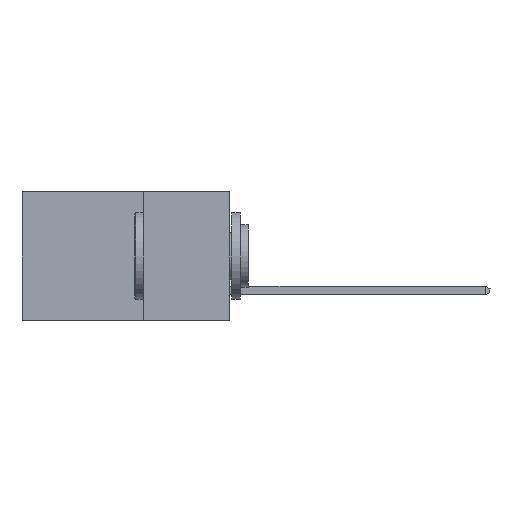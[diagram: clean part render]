
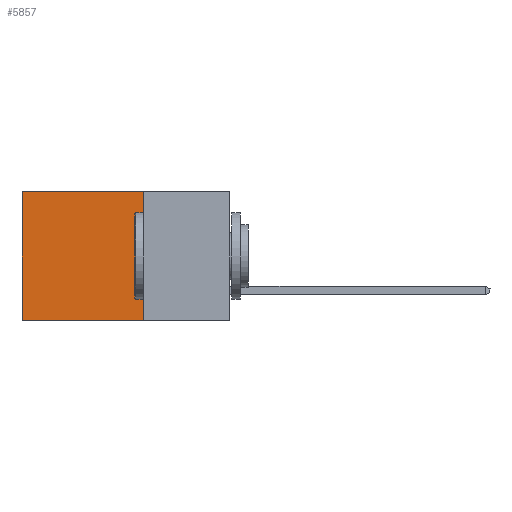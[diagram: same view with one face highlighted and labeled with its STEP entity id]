
A CAD part, left-side view. The second image highlights one B-rep face of the part: STEP entity #5857.
In plain terms, the highlighted planar face has unit normal (-1, 0, 0).
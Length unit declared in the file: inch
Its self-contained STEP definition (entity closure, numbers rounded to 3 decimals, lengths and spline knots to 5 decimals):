
#825 = LINE ( 'NONE', #24037, #21708 ) ;
#930 = LINE ( 'NONE', #24005, #3049 ) ;
#1168 = FACE_OUTER_BOUND ( 'NONE', #21110, .T. ) ;
#3049 = VECTOR ( 'NONE', #10868, 39.37008 ) ;
#3925 = VERTEX_POINT ( 'NONE', #17369 ) ;
#4615 = DIRECTION ( 'NONE',  ( 0., 0., -1. ) ) ;
#5441 = DIRECTION ( 'NONE',  ( 0., 1., 0. ) ) ;
#5582 = EDGE_CURVE ( 'NONE', #18088, #3925, #930, .T. ) ;
#5738 = CARTESIAN_POINT ( 'NONE',  ( 0.2615, 0.25, -0.37 ) ) ;
#5812 = LINE ( 'NONE', #21513, #15614 ) ;
#5857 = ADVANCED_FACE ( 'NONE', ( #1168 ), #14283, .F. ) ;
#6468 = EDGE_CURVE ( 'NONE', #18088, #22148, #21673, .T. ) ;
#6572 = DIRECTION ( 'NONE',  ( 0., 0., -1. ) ) ;
#7212 = VECTOR ( 'NONE', #21308, 39.37008 ) ;
#7704 = ORIENTED_EDGE ( 'NONE', *, *, #5582, .T. ) ;
#7742 = ORIENTED_EDGE ( 'NONE', *, *, #6468, .F. ) ;
#9132 = VERTEX_POINT ( 'NONE', #14184 ) ;
#9231 = ORIENTED_EDGE ( 'NONE', *, *, #25156, .T. ) ;
#10382 = EDGE_CURVE ( 'NONE', #22148, #9132, #5812, .T. ) ;
#10868 = DIRECTION ( 'NONE',  ( 0., 1., 0. ) ) ;
#14184 = CARTESIAN_POINT ( 'NONE',  ( 0.2615, 0.6, -0.37 ) ) ;
#14283 = PLANE ( 'NONE',  #25019 ) ;
#15614 = VECTOR ( 'NONE', #5441, 39.37008 ) ;
#16348 = CARTESIAN_POINT ( 'NONE',  ( 0.2615, 0.25, -0.37 ) ) ;
#17369 = CARTESIAN_POINT ( 'NONE',  ( 0.2615, 0.6, 0. ) ) ;
#17827 = CARTESIAN_POINT ( 'NONE',  ( 0.2615, 0.25, -0.37 ) ) ;
#18088 = VERTEX_POINT ( 'NONE', #18772 ) ;
#18772 = CARTESIAN_POINT ( 'NONE',  ( 0.2615, 0.25, 0. ) ) ;
#21110 = EDGE_LOOP ( 'NONE', ( #9231, #21453, #7742, #7704 ) ) ;
#21308 = DIRECTION ( 'NONE',  ( 0., 0., -1. ) ) ;
#21453 = ORIENTED_EDGE ( 'NONE', *, *, #10382, .F. ) ;
#21513 = CARTESIAN_POINT ( 'NONE',  ( 0.2615, 0.25, -0.37 ) ) ;
#21673 = LINE ( 'NONE', #5738, #7212 ) ;
#21708 = VECTOR ( 'NONE', #6572, 39.37008 ) ;
#22100 = DIRECTION ( 'NONE',  ( 1., 0., 0. ) ) ;
#22148 = VERTEX_POINT ( 'NONE', #17827 ) ;
#24005 = CARTESIAN_POINT ( 'NONE',  ( 0.2615, 0.25, 0. ) ) ;
#24037 = CARTESIAN_POINT ( 'NONE',  ( 0.2615, 0.6, -0.37 ) ) ;
#25019 = AXIS2_PLACEMENT_3D ( 'NONE', #16348, #22100, #4615 ) ;
#25156 = EDGE_CURVE ( 'NONE', #3925, #9132, #825, .T. ) ;
